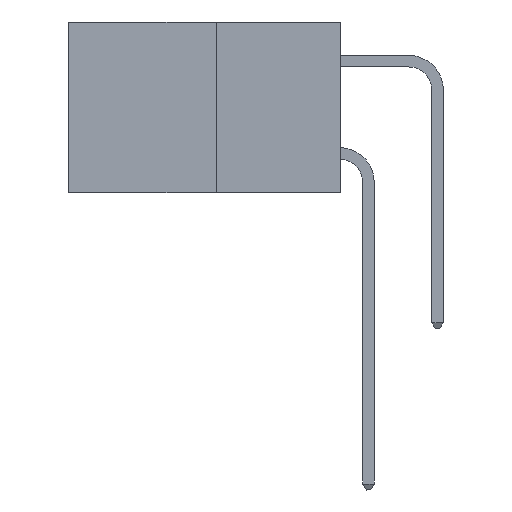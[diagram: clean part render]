
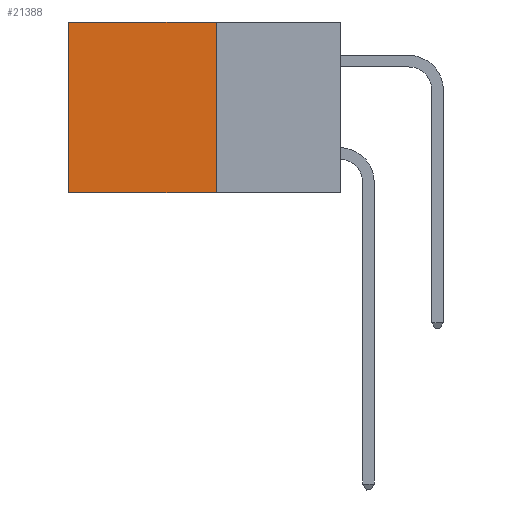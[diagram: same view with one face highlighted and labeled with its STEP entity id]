
A CAD part, left-side view. The second image highlights one B-rep face of the part: STEP entity #21388.
In plain terms, the highlighted planar face has unit normal (-1, 0, 0).
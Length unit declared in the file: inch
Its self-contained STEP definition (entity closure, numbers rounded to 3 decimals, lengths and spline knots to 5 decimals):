
#95 = DIRECTION ( 'NONE',  ( 0., 1., 0. ) ) ;
#1141 = DIRECTION ( 'NONE',  ( 0., 0., -1. ) ) ;
#1623 = VERTEX_POINT ( 'NONE', #6654 ) ;
#2235 = PLANE ( 'NONE',  #11265 ) ;
#2961 = CARTESIAN_POINT ( 'NONE',  ( 0.277, 0.27, -0.37 ) ) ;
#3185 = FACE_OUTER_BOUND ( 'NONE', #20333, .T. ) ;
#3881 = CARTESIAN_POINT ( 'NONE',  ( 0.277, 0.27, -0.37 ) ) ;
#4049 = DIRECTION ( 'NONE',  ( 0., 0., -1. ) ) ;
#4264 = ORIENTED_EDGE ( 'NONE', *, *, #22787, .T. ) ;
#5056 = ORIENTED_EDGE ( 'NONE', *, *, #5492, .F. ) ;
#5492 = EDGE_CURVE ( 'NONE', #1623, #21923, #8279, .T. ) ;
#5755 = CARTESIAN_POINT ( 'NONE',  ( 0.277, 0.27, 0. ) ) ;
#6584 = CARTESIAN_POINT ( 'NONE',  ( 0.277, 0.59, -0.37 ) ) ;
#6654 = CARTESIAN_POINT ( 'NONE',  ( 0.277, 0.27, 0. ) ) ;
#6935 = CARTESIAN_POINT ( 'NONE',  ( 0.277, 0.27, -0.37 ) ) ;
#7519 = DIRECTION ( 'NONE',  ( 0., 1., 0. ) ) ;
#8279 = LINE ( 'NONE', #2961, #17174 ) ;
#9131 = VECTOR ( 'NONE', #19005, 39.37008 ) ;
#11265 = AXIS2_PLACEMENT_3D ( 'NONE', #18200, #14704, #4049 ) ;
#13715 = EDGE_CURVE ( 'NONE', #21923, #19964, #22776, .T. ) ;
#14590 = CARTESIAN_POINT ( 'NONE',  ( 0.277, 0.59, -0.37 ) ) ;
#14704 = DIRECTION ( 'NONE',  ( 1., 0., 0. ) ) ;
#15866 = ORIENTED_EDGE ( 'NONE', *, *, #20342, .T. ) ;
#16125 = ORIENTED_EDGE ( 'NONE', *, *, #13715, .F. ) ;
#17174 = VECTOR ( 'NONE', #1141, 39.37008 ) ;
#17309 = VECTOR ( 'NONE', #7519, 39.37008 ) ;
#17505 = VECTOR ( 'NONE', #95, 39.37008 ) ;
#18200 = CARTESIAN_POINT ( 'NONE',  ( 0.277, 0.27, -0.37 ) ) ;
#19005 = DIRECTION ( 'NONE',  ( 0., 0., -1. ) ) ;
#19964 = VERTEX_POINT ( 'NONE', #14590 ) ;
#20333 = EDGE_LOOP ( 'NONE', ( #15866, #16125, #5056, #4264 ) ) ;
#20342 = EDGE_CURVE ( 'NONE', #21810, #19964, #22743, .T. ) ;
#21388 = ADVANCED_FACE ( 'NONE', ( #3185 ), #2235, .F. ) ;
#21810 = VERTEX_POINT ( 'NONE', #22618 ) ;
#21923 = VERTEX_POINT ( 'NONE', #6935 ) ;
#22580 = LINE ( 'NONE', #5755, #17309 ) ;
#22618 = CARTESIAN_POINT ( 'NONE',  ( 0.277, 0.59, 0. ) ) ;
#22743 = LINE ( 'NONE', #6584, #9131 ) ;
#22776 = LINE ( 'NONE', #3881, #17505 ) ;
#22787 = EDGE_CURVE ( 'NONE', #1623, #21810, #22580, .T. ) ;
